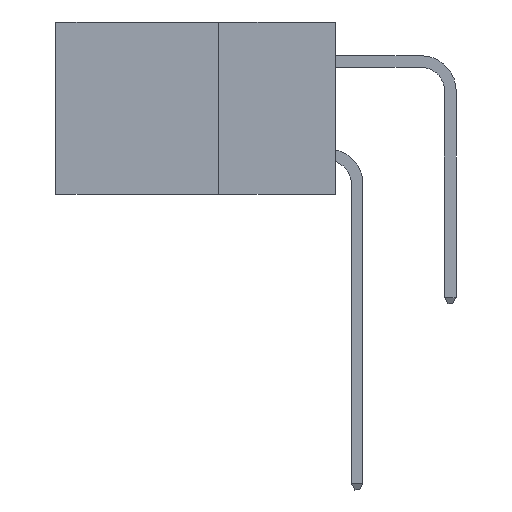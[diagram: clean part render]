
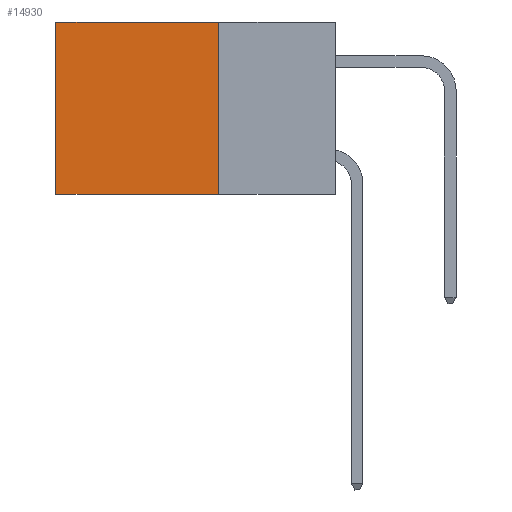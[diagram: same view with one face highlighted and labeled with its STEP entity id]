
A CAD part, left-side view. The second image highlights one B-rep face of the part: STEP entity #14930.
In plain terms, the highlighted planar face has unit normal (-1, 0, 0).
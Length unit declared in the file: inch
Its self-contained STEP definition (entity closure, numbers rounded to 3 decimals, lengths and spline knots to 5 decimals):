
#2866 = VERTEX_POINT ( 'NONE', #11156 ) ;
#2938 = EDGE_CURVE ( 'NONE', #5402, #18184, #12239, .T. ) ;
#2999 = CARTESIAN_POINT ( 'NONE',  ( 0.2875, 0.6, 0. ) ) ;
#3095 = DIRECTION ( 'NONE',  ( 0., 0., -1. ) ) ;
#3815 = FACE_OUTER_BOUND ( 'NONE', #24466, .T. ) ;
#4977 = CARTESIAN_POINT ( 'NONE',  ( 0.2875, 0.6, 0. ) ) ;
#5131 = LINE ( 'NONE', #25976, #24942 ) ;
#5402 = VERTEX_POINT ( 'NONE', #17985 ) ;
#5643 = DIRECTION ( 'NONE',  ( 0., 1., 0. ) ) ;
#6755 = VECTOR ( 'NONE', #23502, 39.37008 ) ;
#6947 = LINE ( 'NONE', #24988, #14381 ) ;
#7632 = ORIENTED_EDGE ( 'NONE', *, *, #10795, .T. ) ;
#8702 = ORIENTED_EDGE ( 'NONE', *, *, #14957, .T. ) ;
#10795 = EDGE_CURVE ( 'NONE', #5402, #16106, #6947, .T. ) ;
#11156 = CARTESIAN_POINT ( 'NONE',  ( 0.2875, 0.6, -0.37 ) ) ;
#11216 = VECTOR ( 'NONE', #23825, 39.37008 ) ;
#12239 = LINE ( 'NONE', #15499, #6755 ) ;
#12572 = AXIS2_PLACEMENT_3D ( 'NONE', #23648, #19584, #3095 ) ;
#12809 = DIRECTION ( 'NONE',  ( 0., 1., 0. ) ) ;
#14381 = VECTOR ( 'NONE', #12809, 39.37008 ) ;
#14612 = ORIENTED_EDGE ( 'NONE', *, *, #2938, .F. ) ;
#14930 = ADVANCED_FACE ( 'NONE', ( #3815 ), #21549, .F. ) ;
#14957 = EDGE_CURVE ( 'NONE', #16106, #2866, #21296, .T. ) ;
#15352 = CARTESIAN_POINT ( 'NONE',  ( 0.2875, 0.25, -0.37 ) ) ;
#15499 = CARTESIAN_POINT ( 'NONE',  ( 0.2875, 0.25, 0. ) ) ;
#16106 = VERTEX_POINT ( 'NONE', #2999 ) ;
#17985 = CARTESIAN_POINT ( 'NONE',  ( 0.2875, 0.25, 0. ) ) ;
#18184 = VERTEX_POINT ( 'NONE', #15352 ) ;
#19584 = DIRECTION ( 'NONE',  ( 1., 0., 0. ) ) ;
#21296 = LINE ( 'NONE', #4977, #11216 ) ;
#21549 = PLANE ( 'NONE',  #12572 ) ;
#23187 = EDGE_CURVE ( 'NONE', #18184, #2866, #5131, .T. ) ;
#23502 = DIRECTION ( 'NONE',  ( 0., 0., -1. ) ) ;
#23648 = CARTESIAN_POINT ( 'NONE',  ( 0.2875, 0.25, 0. ) ) ;
#23825 = DIRECTION ( 'NONE',  ( 0., 0., -1. ) ) ;
#24466 = EDGE_LOOP ( 'NONE', ( #8702, #24602, #14612, #7632 ) ) ;
#24602 = ORIENTED_EDGE ( 'NONE', *, *, #23187, .F. ) ;
#24942 = VECTOR ( 'NONE', #5643, 39.37008 ) ;
#24988 = CARTESIAN_POINT ( 'NONE',  ( 0.2875, 0.25, 0. ) ) ;
#25976 = CARTESIAN_POINT ( 'NONE',  ( 0.2875, 0.25, -0.37 ) ) ;
